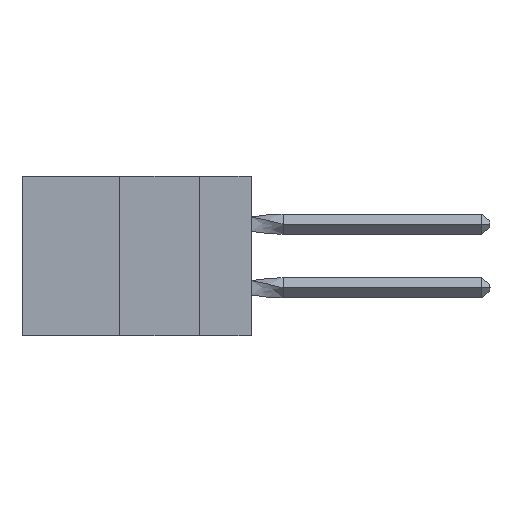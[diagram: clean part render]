
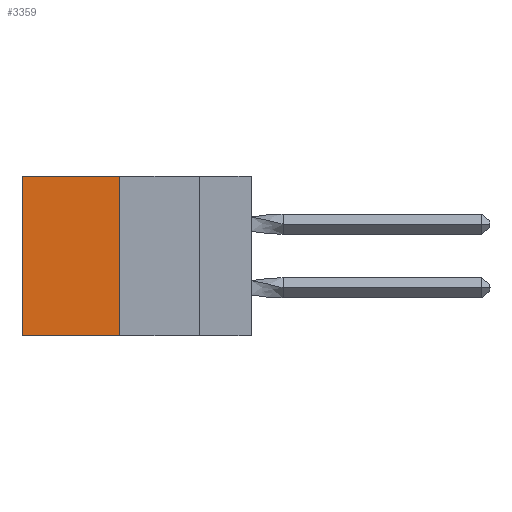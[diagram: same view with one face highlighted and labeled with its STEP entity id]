
A CAD part, left-side view. The second image highlights one B-rep face of the part: STEP entity #3359.
In plain terms, the highlighted planar face has unit normal (-1, 0, 0).
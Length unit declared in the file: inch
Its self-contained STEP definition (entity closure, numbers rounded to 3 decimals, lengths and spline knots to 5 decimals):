
#442 = CARTESIAN_POINT ( 'NONE',  ( 0.305, 0.413, -0.5 ) ) ;
#632 = EDGE_CURVE ( 'NONE', #954, #18134, #14120, .T. ) ;
#954 = VERTEX_POINT ( 'NONE', #6484 ) ;
#974 = VECTOR ( 'NONE', #29429, 39.37008 ) ;
#1621 = VERTEX_POINT ( 'NONE', #26539 ) ;
#2264 = DIRECTION ( 'NONE',  ( 1., 0., 0. ) ) ;
#2728 = VECTOR ( 'NONE', #15319, 39.37008 ) ;
#3359 = ADVANCED_FACE ( 'NONE', ( #20820 ), #24061, .F. ) ;
#3642 = EDGE_CURVE ( 'NONE', #8134, #18134, #8188, .T. ) ;
#6484 = CARTESIAN_POINT ( 'NONE',  ( 0.305, 0.72, 0. ) ) ;
#8134 = VERTEX_POINT ( 'NONE', #10179 ) ;
#8188 = LINE ( 'NONE', #442, #2728 ) ;
#8417 = CARTESIAN_POINT ( 'NONE',  ( 0.305, 0.413, -0.5 ) ) ;
#9303 = CARTESIAN_POINT ( 'NONE',  ( 0.305, 0.413, -0.5 ) ) ;
#9311 = ORIENTED_EDGE ( 'NONE', *, *, #16260, .T. ) ;
#10153 = CARTESIAN_POINT ( 'NONE',  ( 0.305, 0.413, 0. ) ) ;
#10179 = CARTESIAN_POINT ( 'NONE',  ( 0.305, 0.413, -0.5 ) ) ;
#12475 = VECTOR ( 'NONE', #20914, 39.37008 ) ;
#14120 = LINE ( 'NONE', #19432, #19869 ) ;
#15319 = DIRECTION ( 'NONE',  ( 0., 1., 0. ) ) ;
#16260 = EDGE_CURVE ( 'NONE', #1621, #954, #18294, .T. ) ;
#17447 = EDGE_LOOP ( 'NONE', ( #30257, #30922, #25353, #9311 ) ) ;
#18134 = VERTEX_POINT ( 'NONE', #26246 ) ;
#18294 = LINE ( 'NONE', #10153, #974 ) ;
#19069 = DIRECTION ( 'NONE',  ( 0., 0., -1. ) ) ;
#19432 = CARTESIAN_POINT ( 'NONE',  ( 0.305, 0.72, -0.5 ) ) ;
#19869 = VECTOR ( 'NONE', #29417, 39.37008 ) ;
#20820 = FACE_OUTER_BOUND ( 'NONE', #17447, .T. ) ;
#20914 = DIRECTION ( 'NONE',  ( 0., 0., -1. ) ) ;
#24061 = PLANE ( 'NONE',  #30236 ) ;
#25353 = ORIENTED_EDGE ( 'NONE', *, *, #26629, .F. ) ;
#26246 = CARTESIAN_POINT ( 'NONE',  ( 0.305, 0.72, -0.5 ) ) ;
#26539 = CARTESIAN_POINT ( 'NONE',  ( 0.305, 0.413, 0. ) ) ;
#26629 = EDGE_CURVE ( 'NONE', #1621, #8134, #28611, .T. ) ;
#28611 = LINE ( 'NONE', #8417, #12475 ) ;
#29417 = DIRECTION ( 'NONE',  ( 0., 0., -1. ) ) ;
#29429 = DIRECTION ( 'NONE',  ( 0., 1., 0. ) ) ;
#30236 = AXIS2_PLACEMENT_3D ( 'NONE', #9303, #2264, #19069 ) ;
#30257 = ORIENTED_EDGE ( 'NONE', *, *, #632, .T. ) ;
#30922 = ORIENTED_EDGE ( 'NONE', *, *, #3642, .F. ) ;
